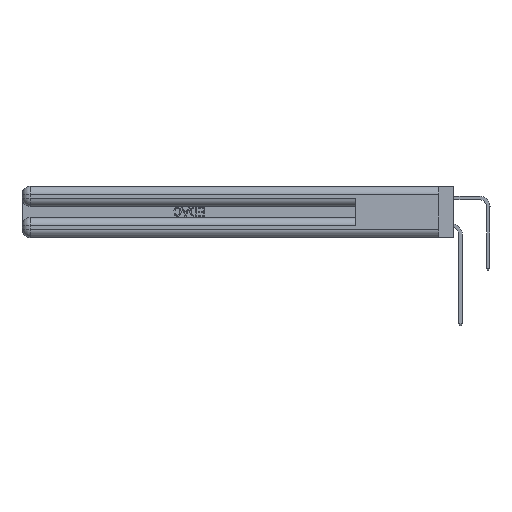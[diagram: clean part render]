
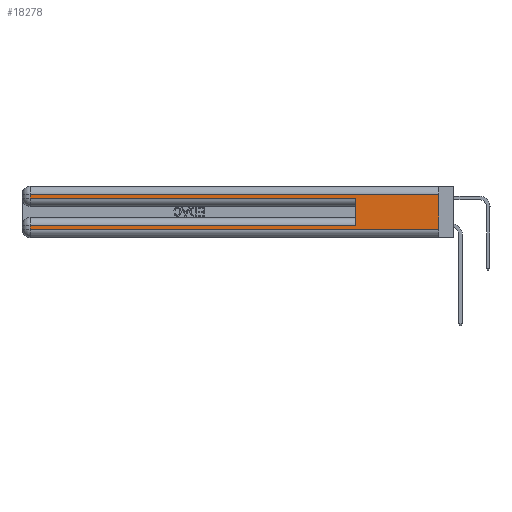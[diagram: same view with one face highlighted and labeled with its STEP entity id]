
A CAD part, left-side view. The second image highlights one B-rep face of the part: STEP entity #18278.
In plain terms, the highlighted planar face has unit normal (-1, 0, 0).
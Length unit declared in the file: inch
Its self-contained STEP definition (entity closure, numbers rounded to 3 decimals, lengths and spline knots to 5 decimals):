
#4090 = VERTEX_POINT ( 'NONE', #22662 ) ;
#4553 = EDGE_CURVE ( 'NONE', #40285, #14963, #4643, .T. ) ;
#4643 = LINE ( 'NONE', #26929, #29987 ) ;
#4866 = LINE ( 'NONE', #18672, #23833 ) ;
#5028 = ORIENTED_EDGE ( 'NONE', *, *, #22384, .T. ) ;
#5102 = VECTOR ( 'NONE', #28445, 39.37008 ) ;
#5510 = DIRECTION ( 'NONE',  ( 1., 0., 0. ) ) ;
#5803 = ORIENTED_EDGE ( 'NONE', *, *, #4553, .F. ) ;
#6250 = DIRECTION ( 'NONE',  ( 0., 0., -1. ) ) ;
#6469 = DIRECTION ( 'NONE',  ( 0., 0., 1. ) ) ;
#6644 = VECTOR ( 'NONE', #18984, 39.37008 ) ;
#6966 = FACE_OUTER_BOUND ( 'NONE', #37014, .T. ) ;
#7239 = EDGE_CURVE ( 'NONE', #23703, #39499, #10593, .T. ) ;
#8126 = CARTESIAN_POINT ( 'NONE',  ( 0., 2.94, 0.37 ) ) ;
#8507 = CARTESIAN_POINT ( 'NONE',  ( 0., 2.94, 0.31 ) ) ;
#8906 = CARTESIAN_POINT ( 'NONE',  ( 0., 0., 0.31 ) ) ;
#9587 = DIRECTION ( 'NONE',  ( 0., -1., 0. ) ) ;
#9825 = LINE ( 'NONE', #15556, #6644 ) ;
#10593 = LINE ( 'NONE', #8126, #20633 ) ;
#13649 = ORIENTED_EDGE ( 'NONE', *, *, #7239, .T. ) ;
#14222 = VECTOR ( 'NONE', #6250, 39.37008 ) ;
#14963 = VERTEX_POINT ( 'NONE', #30589 ) ;
#15108 = LINE ( 'NONE', #39008, #5102 ) ;
#15297 = LINE ( 'NONE', #36696, #14222 ) ;
#15556 = CARTESIAN_POINT ( 'NONE',  ( 0., 0., 0.085 ) ) ;
#18278 = ADVANCED_FACE ( 'NONE', ( #6966 ), #31911, .F. ) ;
#18301 = EDGE_CURVE ( 'NONE', #18311, #23703, #4866, .T. ) ;
#18311 = VERTEX_POINT ( 'NONE', #8906 ) ;
#18672 = CARTESIAN_POINT ( 'NONE',  ( 0., 0., 0.31 ) ) ;
#18984 = DIRECTION ( 'NONE',  ( 0., 1., 0. ) ) ;
#19861 = EDGE_CURVE ( 'NONE', #40285, #4090, #9825, .T. ) ;
#20209 = VECTOR ( 'NONE', #9587, 39.37008 ) ;
#20633 = VECTOR ( 'NONE', #31570, 39.37008 ) ;
#22384 = EDGE_CURVE ( 'NONE', #4090, #27226, #33561, .T. ) ;
#22662 = CARTESIAN_POINT ( 'NONE',  ( 0., 2.94, 0.085 ) ) ;
#23703 = VERTEX_POINT ( 'NONE', #8507 ) ;
#23833 = VECTOR ( 'NONE', #42077, 39.37008 ) ;
#24314 = CARTESIAN_POINT ( 'NONE',  ( 0., 2.94, 0.285 ) ) ;
#25087 = DIRECTION ( 'NONE',  ( 0., 0., -1. ) ) ;
#25842 = ORIENTED_EDGE ( 'NONE', *, *, #18301, .T. ) ;
#26323 = EDGE_CURVE ( 'NONE', #39499, #14963, #15108, .T. ) ;
#26929 = CARTESIAN_POINT ( 'NONE',  ( 0., 0.6, 0.145 ) ) ;
#27226 = VERTEX_POINT ( 'NONE', #32122 ) ;
#27573 = CARTESIAN_POINT ( 'NONE',  ( 0., 0.6, 0.085 ) ) ;
#28445 = DIRECTION ( 'NONE',  ( 0., -1., 0. ) ) ;
#29141 = LINE ( 'NONE', #39466, #20209 ) ;
#29626 = ORIENTED_EDGE ( 'NONE', *, *, #19861, .T. ) ;
#29987 = VECTOR ( 'NONE', #6469, 39.37008 ) ;
#30589 = CARTESIAN_POINT ( 'NONE',  ( 0., 0.6, 0.285 ) ) ;
#31570 = DIRECTION ( 'NONE',  ( 0., 0., -1. ) ) ;
#31911 = PLANE ( 'NONE',  #39248 ) ;
#32122 = CARTESIAN_POINT ( 'NONE',  ( 0., 2.94, 0.06 ) ) ;
#33561 = LINE ( 'NONE', #35990, #42093 ) ;
#33722 = EDGE_CURVE ( 'NONE', #18311, #41627, #15297, .T. ) ;
#34932 = ORIENTED_EDGE ( 'NONE', *, *, #43806, .T. ) ;
#35990 = CARTESIAN_POINT ( 'NONE',  ( 0., 2.94, 0.37 ) ) ;
#36696 = CARTESIAN_POINT ( 'NONE',  ( 0., 0., 0.37 ) ) ;
#36856 = ORIENTED_EDGE ( 'NONE', *, *, #26323, .T. ) ;
#37014 = EDGE_LOOP ( 'NONE', ( #40395, #25842, #13649, #36856, #5803, #29626, #5028, #34932 ) ) ;
#39008 = CARTESIAN_POINT ( 'NONE',  ( 0., 0., 0.285 ) ) ;
#39248 = AXIS2_PLACEMENT_3D ( 'NONE', #42048, #5510, #25087 ) ;
#39466 = CARTESIAN_POINT ( 'NONE',  ( 0., 0., 0.06 ) ) ;
#39499 = VERTEX_POINT ( 'NONE', #24314 ) ;
#39568 = DIRECTION ( 'NONE',  ( 0., 0., -1. ) ) ;
#40285 = VERTEX_POINT ( 'NONE', #27573 ) ;
#40395 = ORIENTED_EDGE ( 'NONE', *, *, #33722, .F. ) ;
#41176 = CARTESIAN_POINT ( 'NONE',  ( 0., 0., 0.06 ) ) ;
#41627 = VERTEX_POINT ( 'NONE', #41176 ) ;
#42048 = CARTESIAN_POINT ( 'NONE',  ( 0., 0., 0.37 ) ) ;
#42077 = DIRECTION ( 'NONE',  ( 0., 1., 0. ) ) ;
#42093 = VECTOR ( 'NONE', #39568, 39.37008 ) ;
#43806 = EDGE_CURVE ( 'NONE', #27226, #41627, #29141, .T. ) ;
